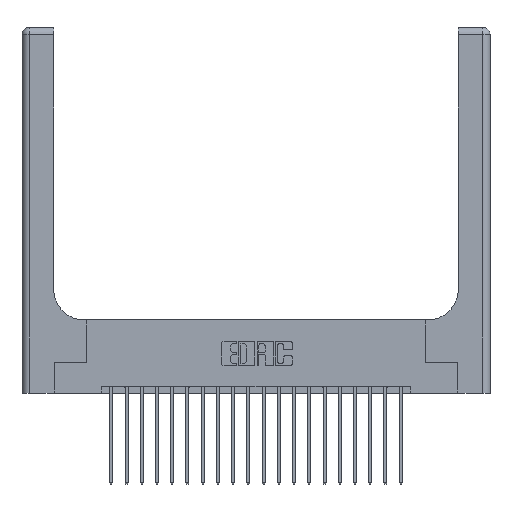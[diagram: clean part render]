
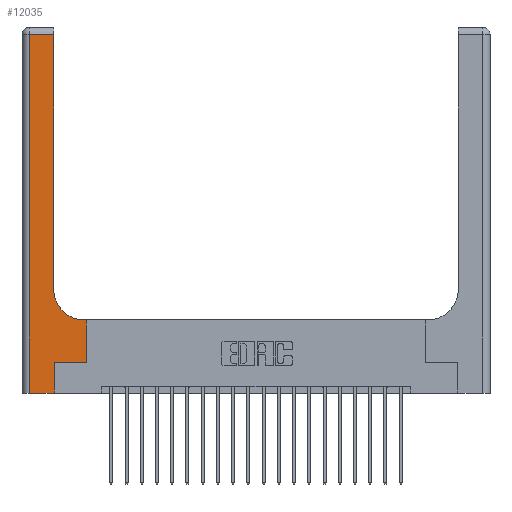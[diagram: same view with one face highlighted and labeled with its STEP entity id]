
A CAD part, top view. The second image highlights one B-rep face of the part: STEP entity #12035.
In plain terms, the highlighted planar face has unit normal (0, 0, 1).
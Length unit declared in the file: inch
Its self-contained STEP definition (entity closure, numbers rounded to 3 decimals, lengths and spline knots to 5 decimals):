
#227 = DIRECTION ( 'NONE',  ( 0., -1., 0. ) ) ;
#1124 = CARTESIAN_POINT ( 'NONE',  ( 0., 3., 0.37 ) ) ;
#1557 = PLANE ( 'NONE',  #14190 ) ;
#1617 = EDGE_CURVE ( 'NONE', #18780, #3454, #9833, .T. ) ;
#1937 = CARTESIAN_POINT ( 'NONE',  ( 0.26, 0.6, 0.37 ) ) ;
#2658 = ORIENTED_EDGE ( 'NONE', *, *, #4166, .T. ) ;
#2745 = VERTEX_POINT ( 'NONE', #15315 ) ;
#2772 = AXIS2_PLACEMENT_3D ( 'NONE', #11493, #18209, #8159 ) ;
#2888 = EDGE_LOOP ( 'NONE', ( #20009, #18734, #2658, #4660, #3775, #13915, #14401, #10116, #6004 ) ) ;
#2952 = DIRECTION ( 'NONE',  ( 0., 1., 0. ) ) ;
#3255 = CARTESIAN_POINT ( 'NONE',  ( 0.265, 0., 0.37 ) ) ;
#3454 = VERTEX_POINT ( 'NONE', #12399 ) ;
#3775 = ORIENTED_EDGE ( 'NONE', *, *, #19281, .T. ) ;
#4166 = EDGE_CURVE ( 'NONE', #14816, #18780, #8226, .T. ) ;
#4180 = VERTEX_POINT ( 'NONE', #11312 ) ;
#4397 = DIRECTION ( 'NONE',  ( 0., 1., 0. ) ) ;
#4660 = ORIENTED_EDGE ( 'NONE', *, *, #1617, .T. ) ;
#4675 = EDGE_CURVE ( 'NONE', #13467, #4180, #20686, .T. ) ;
#5144 = LINE ( 'NONE', #3255, #19023 ) ;
#5509 = EDGE_CURVE ( 'NONE', #20204, #12166, #21184, .T. ) ;
#5511 = VECTOR ( 'NONE', #227, 39.37008 ) ;
#6004 = ORIENTED_EDGE ( 'NONE', *, *, #9471, .T. ) ;
#7385 = DIRECTION ( 'NONE',  ( -1., 0., 0. ) ) ;
#7449 = CARTESIAN_POINT ( 'NONE',  ( 0.26, 0.85, 0.37 ) ) ;
#7709 = DIRECTION ( 'NONE',  ( 1., 0., 0. ) ) ;
#7741 = VECTOR ( 'NONE', #4397, 39.37008 ) ;
#8159 = DIRECTION ( 'NONE',  ( 1., 0., 0. ) ) ;
#8226 = LINE ( 'NONE', #8557, #5511 ) ;
#8367 = DIRECTION ( 'NONE',  ( 1., 0., 0. ) ) ;
#8557 = CARTESIAN_POINT ( 'NONE',  ( 0.06, 3., 0.37 ) ) ;
#8608 = VECTOR ( 'NONE', #7709, 39.37008 ) ;
#9193 = LINE ( 'NONE', #19340, #16918 ) ;
#9471 = EDGE_CURVE ( 'NONE', #14669, #13467, #14051, .T. ) ;
#9677 = DIRECTION ( 'NONE',  ( 0., 1., 0. ) ) ;
#9833 = LINE ( 'NONE', #16555, #8608 ) ;
#9989 = VECTOR ( 'NONE', #8367, 39.37008 ) ;
#10042 = LINE ( 'NONE', #21553, #9989 ) ;
#10114 = CARTESIAN_POINT ( 'NONE',  ( 0.528, 0.6, 0.37 ) ) ;
#10116 = ORIENTED_EDGE ( 'NONE', *, *, #19742, .T. ) ;
#10247 = VECTOR ( 'NONE', #7385, 39.37008 ) ;
#11312 = CARTESIAN_POINT ( 'NONE',  ( 0.26, 2.94, 0.37 ) ) ;
#11493 = CARTESIAN_POINT ( 'NONE',  ( 0.51, 0.85, 0.37 ) ) ;
#11850 = LINE ( 'NONE', #1937, #10247 ) ;
#12035 = ADVANCED_FACE ( 'NONE', ( #20011 ), #1557, .F. ) ;
#12166 = VERTEX_POINT ( 'NONE', #10114 ) ;
#12399 = CARTESIAN_POINT ( 'NONE',  ( 0.265, 0., 0.37 ) ) ;
#12941 = EDGE_CURVE ( 'NONE', #2745, #20204, #10042, .T. ) ;
#13467 = VERTEX_POINT ( 'NONE', #7449 ) ;
#13915 = ORIENTED_EDGE ( 'NONE', *, *, #12941, .T. ) ;
#13960 = EDGE_CURVE ( 'NONE', #4180, #14816, #9193, .T. ) ;
#14051 = CIRCLE ( 'NONE', #2772, 0.25 ) ;
#14190 = AXIS2_PLACEMENT_3D ( 'NONE', #1124, #19602, #14968 ) ;
#14401 = ORIENTED_EDGE ( 'NONE', *, *, #5509, .T. ) ;
#14669 = VERTEX_POINT ( 'NONE', #19965 ) ;
#14816 = VERTEX_POINT ( 'NONE', #18990 ) ;
#14968 = DIRECTION ( 'NONE',  ( -1., 0., 0. ) ) ;
#15315 = CARTESIAN_POINT ( 'NONE',  ( 0.265, 0.25, 0.37 ) ) ;
#15361 = VECTOR ( 'NONE', #9677, 39.37008 ) ;
#15934 = DIRECTION ( 'NONE',  ( -1., 0., 0. ) ) ;
#16389 = CARTESIAN_POINT ( 'NONE',  ( 0.528, 0.25, 0.37 ) ) ;
#16521 = CARTESIAN_POINT ( 'NONE',  ( 0.06, 0., 0.37 ) ) ;
#16555 = CARTESIAN_POINT ( 'NONE',  ( 0., 0., 0.37 ) ) ;
#16918 = VECTOR ( 'NONE', #15934, 39.37008 ) ;
#18209 = DIRECTION ( 'NONE',  ( 0., 0., -1. ) ) ;
#18734 = ORIENTED_EDGE ( 'NONE', *, *, #13960, .T. ) ;
#18780 = VERTEX_POINT ( 'NONE', #16521 ) ;
#18990 = CARTESIAN_POINT ( 'NONE',  ( 0.06, 2.94, 0.37 ) ) ;
#19023 = VECTOR ( 'NONE', #2952, 39.37008 ) ;
#19072 = CARTESIAN_POINT ( 'NONE',  ( 0.26, 3., 0.37 ) ) ;
#19281 = EDGE_CURVE ( 'NONE', #3454, #2745, #5144, .T. ) ;
#19340 = CARTESIAN_POINT ( 'NONE',  ( 0., 2.94, 0.37 ) ) ;
#19579 = CARTESIAN_POINT ( 'NONE',  ( 0.528, 0.25, 0.37 ) ) ;
#19602 = DIRECTION ( 'NONE',  ( 0., 0., -1. ) ) ;
#19742 = EDGE_CURVE ( 'NONE', #12166, #14669, #11850, .T. ) ;
#19965 = CARTESIAN_POINT ( 'NONE',  ( 0.51, 0.6, 0.37 ) ) ;
#20009 = ORIENTED_EDGE ( 'NONE', *, *, #4675, .T. ) ;
#20011 = FACE_OUTER_BOUND ( 'NONE', #2888, .T. ) ;
#20204 = VERTEX_POINT ( 'NONE', #16389 ) ;
#20686 = LINE ( 'NONE', #19072, #15361 ) ;
#21184 = LINE ( 'NONE', #19579, #7741 ) ;
#21553 = CARTESIAN_POINT ( 'NONE',  ( 0.265, 0.25, 0.37 ) ) ;
